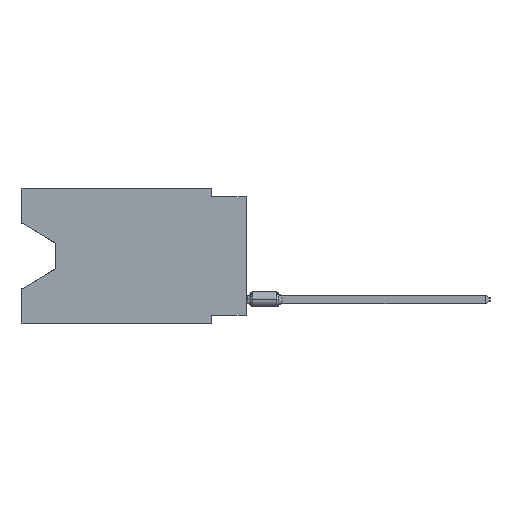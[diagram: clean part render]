
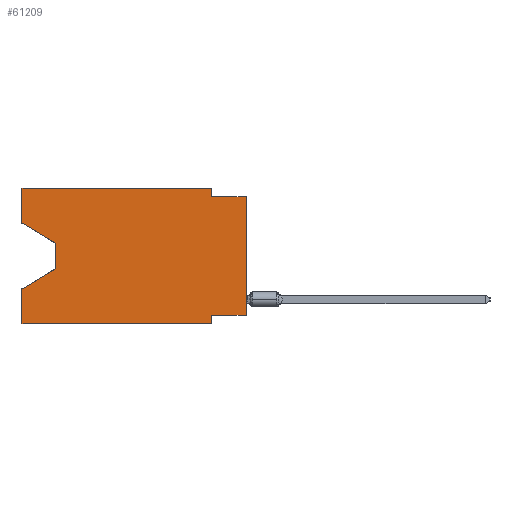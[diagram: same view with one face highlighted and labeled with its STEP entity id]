
A CAD part, left-side view. The second image highlights one B-rep face of the part: STEP entity #61209.
In plain terms, the highlighted planar face has unit normal (-1, 0, 0).
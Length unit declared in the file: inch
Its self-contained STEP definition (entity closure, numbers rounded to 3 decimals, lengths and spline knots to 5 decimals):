
#336 = CARTESIAN_POINT ( 'NONE',  ( 0., 0.1, -0.365 ) ) ;
#989 = CARTESIAN_POINT ( 'NONE',  ( 0., 0.1, -0.39 ) ) ;
#2857 = LINE ( 'NONE', #46967, #17753 ) ;
#3292 = EDGE_CURVE ( 'NONE', #12012, #18360, #2857, .T. ) ;
#3655 = EDGE_CURVE ( 'NONE', #53087, #27664, #12749, .T. ) ;
#4436 = LINE ( 'NONE', #37152, #67036 ) ;
#4621 = VECTOR ( 'NONE', #33277, 39.37008 ) ;
#5270 = ORIENTED_EDGE ( 'NONE', *, *, #50986, .F. ) ;
#5615 = ORIENTED_EDGE ( 'NONE', *, *, #60266, .T. ) ;
#5662 = DIRECTION ( 'NONE',  ( 0., 1., 0. ) ) ;
#7865 = CARTESIAN_POINT ( 'NONE',  ( 0., 0., -0.365 ) ) ;
#8253 = EDGE_CURVE ( 'NONE', #39120, #51701, #15627, .T. ) ;
#8332 = EDGE_CURVE ( 'NONE', #34060, #39120, #59688, .T. ) ;
#8881 = EDGE_CURVE ( 'NONE', #34060, #13319, #48944, .T. ) ;
#9557 = DIRECTION ( 'NONE',  ( 0., 0., -1. ) ) ;
#10604 = DIRECTION ( 'NONE',  ( 0., 0., 1. ) ) ;
#11347 = CARTESIAN_POINT ( 'NONE',  ( 0., 0.645, -0.39 ) ) ;
#12012 = VERTEX_POINT ( 'NONE', #51592 ) ;
#12697 = VERTEX_POINT ( 'NONE', #44955 ) ;
#12749 = LINE ( 'NONE', #22029, #57665 ) ;
#13319 = VERTEX_POINT ( 'NONE', #58342 ) ;
#13368 = VERTEX_POINT ( 'NONE', #11347 ) ;
#14138 = LINE ( 'NONE', #68881, #59060 ) ;
#15627 = LINE ( 'NONE', #30300, #34237 ) ;
#17362 = LINE ( 'NONE', #989, #50990 ) ;
#17523 = EDGE_CURVE ( 'NONE', #12697, #12012, #63275, .T. ) ;
#17753 = VECTOR ( 'NONE', #24551, 39.37008 ) ;
#18360 = VERTEX_POINT ( 'NONE', #48337 ) ;
#19165 = LINE ( 'NONE', #40838, #54139 ) ;
#19473 = VECTOR ( 'NONE', #49031, 39.37008 ) ;
#20423 = FACE_OUTER_BOUND ( 'NONE', #37805, .T. ) ;
#21470 = PLANE ( 'NONE',  #54569 ) ;
#22029 = CARTESIAN_POINT ( 'NONE',  ( 0., 0., -0.365 ) ) ;
#22692 = DIRECTION ( 'NONE',  ( 0., 0., -1. ) ) ;
#24551 = DIRECTION ( 'NONE',  ( 0., -1., 0. ) ) ;
#26123 = DIRECTION ( 'NONE',  ( 0., 0.855, -0.519 ) ) ;
#26380 = VECTOR ( 'NONE', #26732, 39.37008 ) ;
#26382 = CARTESIAN_POINT ( 'NONE',  ( 0., 0.645, -0.39 ) ) ;
#26732 = DIRECTION ( 'NONE',  ( 0., -1., 0. ) ) ;
#27145 = CARTESIAN_POINT ( 'NONE',  ( 0., 0.645, 0. ) ) ;
#27664 = VERTEX_POINT ( 'NONE', #336 ) ;
#28322 = VECTOR ( 'NONE', #9557, 39.37008 ) ;
#28527 = VERTEX_POINT ( 'NONE', #55909 ) ;
#29790 = ORIENTED_EDGE ( 'NONE', *, *, #3292, .F. ) ;
#30300 = CARTESIAN_POINT ( 'NONE',  ( 0., 0.55, -0.158 ) ) ;
#31625 = CARTESIAN_POINT ( 'NONE',  ( 0., 0., 0. ) ) ;
#31945 = EDGE_CURVE ( 'NONE', #13368, #46218, #19165, .T. ) ;
#33277 = DIRECTION ( 'NONE',  ( 0., 0., 1. ) ) ;
#34060 = VERTEX_POINT ( 'NONE', #48715 ) ;
#34237 = VECTOR ( 'NONE', #57697, 39.37008 ) ;
#37152 = CARTESIAN_POINT ( 'NONE',  ( 0., 0.55, -0.232 ) ) ;
#37805 = EDGE_LOOP ( 'NONE', ( #48902, #44781, #49580, #50773, #47428, #5270, #57750, #5615, #29790, #42738, #41445, #55515 ) ) ;
#38041 = EDGE_CURVE ( 'NONE', #13319, #12697, #14138, .T. ) ;
#38775 = VECTOR ( 'NONE', #10604, 39.37008 ) ;
#38929 = EDGE_CURVE ( 'NONE', #13368, #28527, #48436, .T. ) ;
#38945 = CARTESIAN_POINT ( 'NONE',  ( 0., 0.645, 0. ) ) ;
#39120 = VERTEX_POINT ( 'NONE', #49842 ) ;
#40838 = CARTESIAN_POINT ( 'NONE',  ( 0., 0.645, 0. ) ) ;
#41445 = ORIENTED_EDGE ( 'NONE', *, *, #38041, .F. ) ;
#42094 = DIRECTION ( 'NONE',  ( 1., 0., 0. ) ) ;
#42738 = ORIENTED_EDGE ( 'NONE', *, *, #17523, .F. ) ;
#44781 = ORIENTED_EDGE ( 'NONE', *, *, #8253, .T. ) ;
#44955 = CARTESIAN_POINT ( 'NONE',  ( 0., 0.1, 0. ) ) ;
#46218 = VERTEX_POINT ( 'NONE', #65542 ) ;
#46967 = CARTESIAN_POINT ( 'NONE',  ( 0., 0., -0.025 ) ) ;
#47428 = ORIENTED_EDGE ( 'NONE', *, *, #38929, .T. ) ;
#48337 = CARTESIAN_POINT ( 'NONE',  ( 0., 0., -0.025 ) ) ;
#48436 = LINE ( 'NONE', #26382, #26380 ) ;
#48715 = CARTESIAN_POINT ( 'NONE',  ( 0., 0.645, -0.10025 ) ) ;
#48902 = ORIENTED_EDGE ( 'NONE', *, *, #8332, .T. ) ;
#48944 = LINE ( 'NONE', #38945, #4621 ) ;
#49031 = DIRECTION ( 'NONE',  ( 0., -0.855, -0.519 ) ) ;
#49580 = ORIENTED_EDGE ( 'NONE', *, *, #52826, .T. ) ;
#49842 = CARTESIAN_POINT ( 'NONE',  ( 0., 0.55, -0.158 ) ) ;
#50773 = ORIENTED_EDGE ( 'NONE', *, *, #31945, .F. ) ;
#50986 = EDGE_CURVE ( 'NONE', #27664, #28527, #17362, .T. ) ;
#50990 = VECTOR ( 'NONE', #22692, 39.37008 ) ;
#51592 = CARTESIAN_POINT ( 'NONE',  ( 0., 0.1, -0.025 ) ) ;
#51701 = VERTEX_POINT ( 'NONE', #67567 ) ;
#52189 = DIRECTION ( 'NONE',  ( 0., -1., 0. ) ) ;
#52826 = EDGE_CURVE ( 'NONE', #51701, #46218, #4436, .T. ) ;
#52962 = CARTESIAN_POINT ( 'NONE',  ( 0., 0.1, 0. ) ) ;
#53087 = VERTEX_POINT ( 'NONE', #7865 ) ;
#54139 = VECTOR ( 'NONE', #62885, 39.37008 ) ;
#54170 = DIRECTION ( 'NONE',  ( 0., 0., -1. ) ) ;
#54569 = AXIS2_PLACEMENT_3D ( 'NONE', #27145, #42094, #54170 ) ;
#55515 = ORIENTED_EDGE ( 'NONE', *, *, #8881, .F. ) ;
#55909 = CARTESIAN_POINT ( 'NONE',  ( 0., 0.1, -0.39 ) ) ;
#57665 = VECTOR ( 'NONE', #5662, 39.37008 ) ;
#57697 = DIRECTION ( 'NONE',  ( 0., 0., -1. ) ) ;
#57750 = ORIENTED_EDGE ( 'NONE', *, *, #3655, .F. ) ;
#58342 = CARTESIAN_POINT ( 'NONE',  ( 0., 0.645, 0. ) ) ;
#59015 = CARTESIAN_POINT ( 'NONE',  ( 0., 0.645, -0.10025 ) ) ;
#59060 = VECTOR ( 'NONE', #52189, 39.37008 ) ;
#59688 = LINE ( 'NONE', #59015, #19473 ) ;
#60266 = EDGE_CURVE ( 'NONE', #53087, #18360, #69654, .T. ) ;
#61209 = ADVANCED_FACE ( 'NONE', ( #20423 ), #21470, .F. ) ;
#62885 = DIRECTION ( 'NONE',  ( 0., 0., 1. ) ) ;
#63275 = LINE ( 'NONE', #52962, #28322 ) ;
#65542 = CARTESIAN_POINT ( 'NONE',  ( 0., 0.645, -0.28975 ) ) ;
#67036 = VECTOR ( 'NONE', #26123, 39.37008 ) ;
#67567 = CARTESIAN_POINT ( 'NONE',  ( 0., 0.55, -0.232 ) ) ;
#68881 = CARTESIAN_POINT ( 'NONE',  ( 0., 0.645, 0. ) ) ;
#69654 = LINE ( 'NONE', #31625, #38775 ) ;
